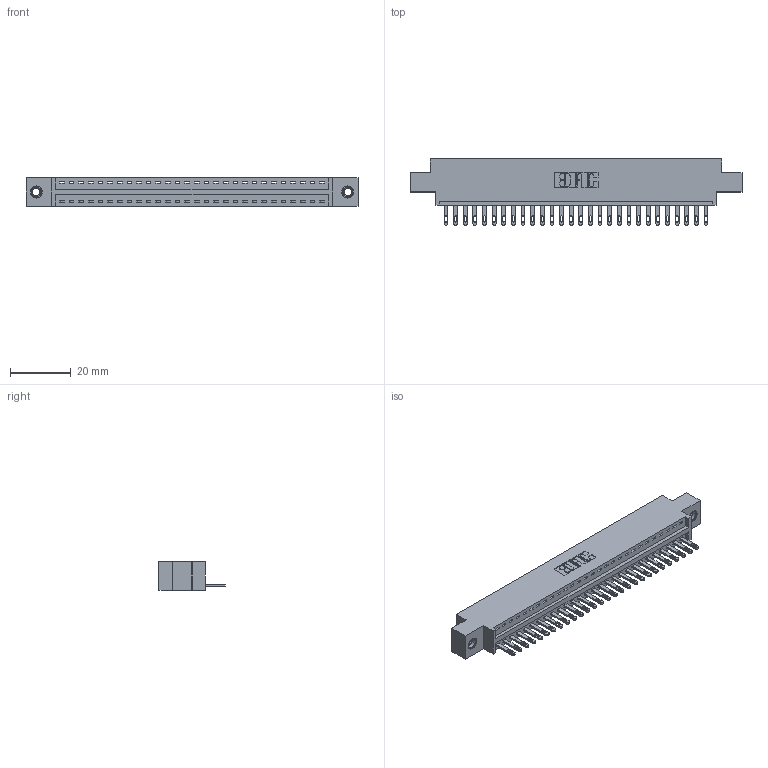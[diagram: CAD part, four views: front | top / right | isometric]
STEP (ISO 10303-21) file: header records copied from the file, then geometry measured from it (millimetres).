
FILE_DESCRIPTION (( 'STEP AP203' ), '1' );
FILE_NAME ('896-028-500-607.STEP', '2021-07-27T18:25:12', ( '' ), ( '' ), 'SwSTEP 2.0', 'SolidWorks 2020', '' );
FILE_SCHEMA (( 'CONFIG_CONTROL_DESIGN' ));
Length unit declared in the file: inch
Products named in the file (4): 896-028-500-607; 345-250-001_345-250-005-103; 345-292-001_345-293-100; 846 Part_0.170 Offset - 0.156 Dia-TI
Assembly tree (31 placements, depth 2):
  896-028-500-607
    846 Part_0.170 Offset - 0.156 Dia-TI
    345-292-001_345-293-100  x28
    345-250-001_345-250-005-103  x2
Bounding box: 109.47 x 21.84 x 9.4 mm (x, y, z)
Volume: 10231.8 mm3; surface area: 12897.6 mm2
Topology: 31 solids, 31 shells, 1698 faces, 5181 edges, 3446 vertices
Faces by surface type: plane 1064, cylinder 618, cone 12, torus 4
Entity records: 20510 total; most frequent: CARTESIAN_POINT 3503, ORIENTED_EDGE 3458, DIRECTION 3135, EDGE_CURVE 1729, LINE 1461, VECTOR 1461, VERTEX_POINT 1148, AXIS2_PLACEMENT_3D 837
